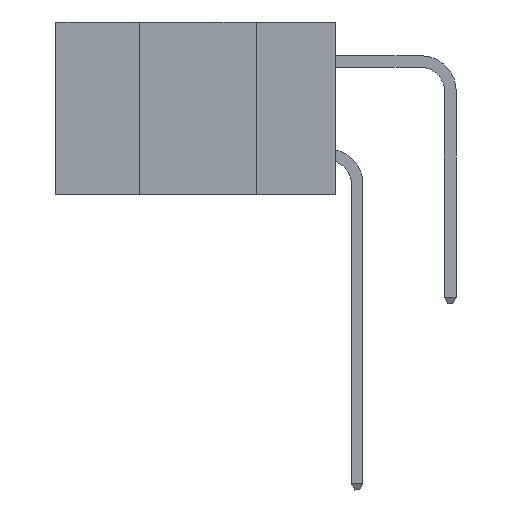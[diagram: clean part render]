
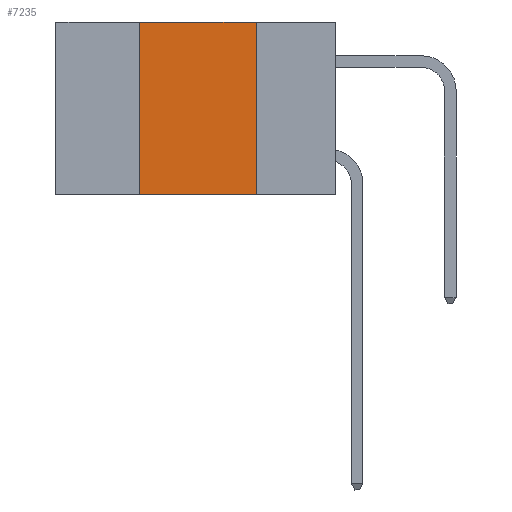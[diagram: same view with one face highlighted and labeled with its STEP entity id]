
A CAD part, left-side view. The second image highlights one B-rep face of the part: STEP entity #7235.
In plain terms, the highlighted planar face has unit normal (-1, 0, 0).
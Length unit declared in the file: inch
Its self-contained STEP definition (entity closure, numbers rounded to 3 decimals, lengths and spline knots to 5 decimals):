
#315 = ORIENTED_EDGE ( 'NONE', *, *, #37758, .T. ) ;
#577 = CARTESIAN_POINT ( 'NONE',  ( 0., 0.17, 0. ) ) ;
#1316 = VERTEX_POINT ( 'NONE', #35002 ) ;
#2008 = CARTESIAN_POINT ( 'NONE',  ( 0., 0.42, 0. ) ) ;
#2806 = ORIENTED_EDGE ( 'NONE', *, *, #27771, .F. ) ;
#2875 = ORIENTED_EDGE ( 'NONE', *, *, #5366, .F. ) ;
#4835 = VERTEX_POINT ( 'NONE', #34825 ) ;
#4966 = DIRECTION ( 'NONE',  ( 0., 0., 1. ) ) ;
#5366 = EDGE_CURVE ( 'NONE', #36193, #4835, #28180, .T. ) ;
#7130 = CARTESIAN_POINT ( 'NONE',  ( 0., 0.17, -0.37 ) ) ;
#7235 = ADVANCED_FACE ( 'NONE', ( #25983 ), #34925, .F. ) ;
#7493 = LINE ( 'NONE', #34317, #31075 ) ;
#9023 = CARTESIAN_POINT ( 'NONE',  ( 0., 0.6, -0.37 ) ) ;
#9723 = LINE ( 'NONE', #577, #17299 ) ;
#10111 = DIRECTION ( 'NONE',  ( 0., 0., -1. ) ) ;
#13319 = VECTOR ( 'NONE', #34575, 39.37008 ) ;
#14114 = DIRECTION ( 'NONE',  ( 0., 0., -1. ) ) ;
#14159 = EDGE_CURVE ( 'NONE', #1316, #36193, #7493, .T. ) ;
#16737 = EDGE_LOOP ( 'NONE', ( #2806, #2875, #25182, #315 ) ) ;
#17155 = AXIS2_PLACEMENT_3D ( 'NONE', #26366, #19960, #14114 ) ;
#17299 = VECTOR ( 'NONE', #10111, 39.37008 ) ;
#19631 = VERTEX_POINT ( 'NONE', #7130 ) ;
#19960 = DIRECTION ( 'NONE',  ( 1., 0., 0. ) ) ;
#22739 = CARTESIAN_POINT ( 'NONE',  ( 0., 0.6, 0. ) ) ;
#25182 = ORIENTED_EDGE ( 'NONE', *, *, #14159, .F. ) ;
#25983 = FACE_OUTER_BOUND ( 'NONE', #16737, .T. ) ;
#26366 = CARTESIAN_POINT ( 'NONE',  ( 0., 0.6, 0. ) ) ;
#26901 = LINE ( 'NONE', #9023, #28389 ) ;
#27771 = EDGE_CURVE ( 'NONE', #4835, #19631, #9723, .T. ) ;
#28180 = LINE ( 'NONE', #22739, #13319 ) ;
#28389 = VECTOR ( 'NONE', #33294, 39.37008 ) ;
#31075 = VECTOR ( 'NONE', #4966, 39.37008 ) ;
#33294 = DIRECTION ( 'NONE',  ( 0., -1., 0. ) ) ;
#34317 = CARTESIAN_POINT ( 'NONE',  ( 0., 0.42, 0. ) ) ;
#34575 = DIRECTION ( 'NONE',  ( 0., -1., 0. ) ) ;
#34825 = CARTESIAN_POINT ( 'NONE',  ( 0., 0.17, 0. ) ) ;
#34925 = PLANE ( 'NONE',  #17155 ) ;
#35002 = CARTESIAN_POINT ( 'NONE',  ( 0., 0.42, -0.37 ) ) ;
#36193 = VERTEX_POINT ( 'NONE', #2008 ) ;
#37758 = EDGE_CURVE ( 'NONE', #1316, #19631, #26901, .T. ) ;
